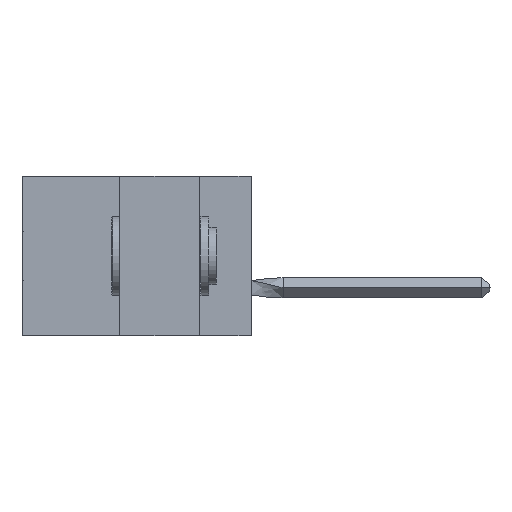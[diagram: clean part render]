
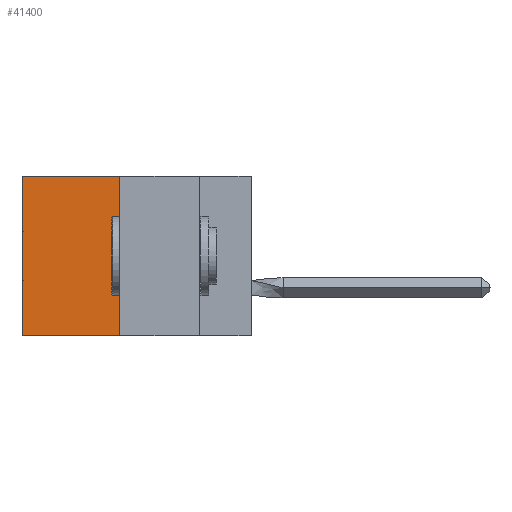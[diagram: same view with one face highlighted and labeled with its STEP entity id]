
A CAD part, left-side view. The second image highlights one B-rep face of the part: STEP entity #41400.
In plain terms, the highlighted planar face has unit normal (-1, 0, 0).
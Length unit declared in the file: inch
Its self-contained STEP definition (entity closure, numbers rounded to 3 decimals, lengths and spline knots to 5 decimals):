
#1323 = ORIENTED_EDGE ( 'NONE', *, *, #3947, .F. ) ;
#2876 = FACE_OUTER_BOUND ( 'NONE', #4525, .T. ) ;
#3947 = EDGE_CURVE ( 'NONE', #16650, #43809, #4248, .T. ) ;
#4248 = LINE ( 'NONE', #23312, #7530 ) ;
#4290 = DIRECTION ( 'NONE',  ( 0., 0., -1. ) ) ;
#4525 = EDGE_LOOP ( 'NONE', ( #37404, #1323, #24164, #8558 ) ) ;
#6002 = CARTESIAN_POINT ( 'NONE',  ( 0.305, 0.413, 0. ) ) ;
#6991 = VERTEX_POINT ( 'NONE', #22201 ) ;
#7499 = CARTESIAN_POINT ( 'NONE',  ( 0.305, 0.72, -0.5 ) ) ;
#7530 = VECTOR ( 'NONE', #40547, 39.37008 ) ;
#8558 = ORIENTED_EDGE ( 'NONE', *, *, #36126, .T. ) ;
#10013 = CARTESIAN_POINT ( 'NONE',  ( 0.305, 0.413, 0. ) ) ;
#13516 = DIRECTION ( 'NONE',  ( 0., 1., 0. ) ) ;
#15676 = AXIS2_PLACEMENT_3D ( 'NONE', #32661, #32962, #19252 ) ;
#16650 = VERTEX_POINT ( 'NONE', #19237 ) ;
#17592 = VECTOR ( 'NONE', #4290, 39.37008 ) ;
#19237 = CARTESIAN_POINT ( 'NONE',  ( 0.305, 0.413, -0.5 ) ) ;
#19252 = DIRECTION ( 'NONE',  ( 0., 0., -1. ) ) ;
#19788 = CARTESIAN_POINT ( 'NONE',  ( 0.305, 0.413, -0.5 ) ) ;
#22201 = CARTESIAN_POINT ( 'NONE',  ( 0.305, 0.72, 0. ) ) ;
#22455 = VERTEX_POINT ( 'NONE', #6002 ) ;
#22895 = CARTESIAN_POINT ( 'NONE',  ( 0.305, 0.72, -0.5 ) ) ;
#23312 = CARTESIAN_POINT ( 'NONE',  ( 0.305, 0.413, -0.5 ) ) ;
#23931 = LINE ( 'NONE', #10013, #26080 ) ;
#24164 = ORIENTED_EDGE ( 'NONE', *, *, #26721, .F. ) ;
#24564 = VECTOR ( 'NONE', #26403, 39.37008 ) ;
#25890 = PLANE ( 'NONE',  #15676 ) ;
#26080 = VECTOR ( 'NONE', #13516, 39.37008 ) ;
#26403 = DIRECTION ( 'NONE',  ( 0., 0., -1. ) ) ;
#26721 = EDGE_CURVE ( 'NONE', #22455, #16650, #34822, .T. ) ;
#30011 = LINE ( 'NONE', #7499, #17592 ) ;
#32661 = CARTESIAN_POINT ( 'NONE',  ( 0.305, 0.413, -0.5 ) ) ;
#32962 = DIRECTION ( 'NONE',  ( 1., 0., 0. ) ) ;
#33656 = EDGE_CURVE ( 'NONE', #6991, #43809, #30011, .T. ) ;
#34822 = LINE ( 'NONE', #19788, #24564 ) ;
#36126 = EDGE_CURVE ( 'NONE', #22455, #6991, #23931, .T. ) ;
#37404 = ORIENTED_EDGE ( 'NONE', *, *, #33656, .T. ) ;
#40547 = DIRECTION ( 'NONE',  ( 0., 1., 0. ) ) ;
#41400 = ADVANCED_FACE ( 'NONE', ( #2876 ), #25890, .F. ) ;
#43809 = VERTEX_POINT ( 'NONE', #22895 ) ;
